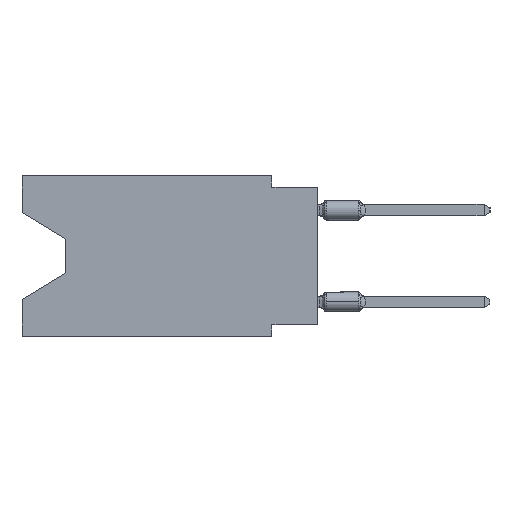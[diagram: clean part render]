
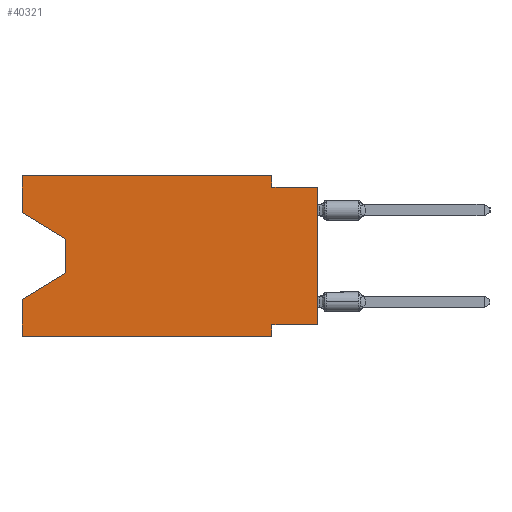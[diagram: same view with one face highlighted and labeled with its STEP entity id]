
A CAD part, left-side view. The second image highlights one B-rep face of the part: STEP entity #40321.
In plain terms, the highlighted planar face has unit normal (-1, 0, 0).
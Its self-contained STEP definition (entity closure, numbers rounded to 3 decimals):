
#712 = CARTESIAN_POINT ( 'NONE',  ( 0., 16.383, 0. ) ) ;
#977 = DIRECTION ( 'NONE',  ( 0., 0., 1. ) ) ;
#1176 = DIRECTION ( 'NONE',  ( 0., 0., -1. ) ) ;
#2780 = ORIENTED_EDGE ( 'NONE', *, *, #12342, .F. ) ;
#3453 = LINE ( 'NONE', #26692, #42703 ) ;
#3868 = CARTESIAN_POINT ( 'NONE',  ( 0., 13.97, -5.385 ) ) ;
#5465 = VERTEX_POINT ( 'NONE', #31540 ) ;
#5962 = VERTEX_POINT ( 'NONE', #16801 ) ;
#6063 = CARTESIAN_POINT ( 'NONE',  ( 0., 13.97, -3.505 ) ) ;
#6569 = LINE ( 'NONE', #40933, #33076 ) ;
#7921 = VECTOR ( 'NONE', #21574, 1000. ) ;
#8168 = DIRECTION ( 'NONE',  ( 0., -1., 0. ) ) ;
#9610 = VERTEX_POINT ( 'NONE', #15506 ) ;
#9838 = CARTESIAN_POINT ( 'NONE',  ( 0., 0., 0. ) ) ;
#9855 = DIRECTION ( 'NONE',  ( 0., 0., -1. ) ) ;
#9978 = LINE ( 'NONE', #25386, #7921 ) ;
#10222 = DIRECTION ( 'NONE',  ( 1., 0., 0. ) ) ;
#10704 = CARTESIAN_POINT ( 'NONE',  ( 0., 16.383, -8.89 ) ) ;
#11739 = VECTOR ( 'NONE', #8168, 1000. ) ;
#12045 = CARTESIAN_POINT ( 'NONE',  ( 0., 2.54, 0. ) ) ;
#12142 = CARTESIAN_POINT ( 'NONE',  ( 0., 16.383, -6.852 ) ) ;
#12342 = EDGE_CURVE ( 'NONE', #37248, #43170, #27362, .T. ) ;
#13881 = DIRECTION ( 'NONE',  ( 0., 0., 1. ) ) ;
#13892 = DIRECTION ( 'NONE',  ( 0., -0.855, -0.519 ) ) ;
#14019 = PLANE ( 'NONE',  #37804 ) ;
#14263 = FACE_OUTER_BOUND ( 'NONE', #23722, .T. ) ;
#14322 = EDGE_CURVE ( 'NONE', #17885, #20145, #6569, .T. ) ;
#14753 = ORIENTED_EDGE ( 'NONE', *, *, #25985, .T. ) ;
#15059 = EDGE_CURVE ( 'NONE', #43170, #9610, #46410, .T. ) ;
#15506 = CARTESIAN_POINT ( 'NONE',  ( 0., 2.54, -0.635 ) ) ;
#15628 = ORIENTED_EDGE ( 'NONE', *, *, #21421, .F. ) ;
#16246 = CARTESIAN_POINT ( 'NONE',  ( 0., 16.383, 0. ) ) ;
#16681 = DIRECTION ( 'NONE',  ( 0., 0., 1. ) ) ;
#16801 = CARTESIAN_POINT ( 'NONE',  ( 0., 16.383, -2.038 ) ) ;
#16958 = VECTOR ( 'NONE', #13892, 1000. ) ;
#17779 = LINE ( 'NONE', #10704, #24912 ) ;
#17885 = VERTEX_POINT ( 'NONE', #32952 ) ;
#18074 = EDGE_CURVE ( 'NONE', #42137, #5465, #17779, .T. ) ;
#19917 = LINE ( 'NONE', #712, #46518 ) ;
#20145 = VERTEX_POINT ( 'NONE', #23142 ) ;
#20218 = LINE ( 'NONE', #39437, #48343 ) ;
#20871 = ORIENTED_EDGE ( 'NONE', *, *, #38188, .F. ) ;
#21421 = EDGE_CURVE ( 'NONE', #9610, #41717, #26017, .T. ) ;
#21574 = DIRECTION ( 'NONE',  ( 0., 0.855, -0.519 ) ) ;
#21725 = CARTESIAN_POINT ( 'NONE',  ( 0., 2.54, 0. ) ) ;
#23142 = CARTESIAN_POINT ( 'NONE',  ( 0., 2.54, -8.255 ) ) ;
#23722 = EDGE_LOOP ( 'NONE', ( #14753, #25947, #23915, #25360, #29523, #34933, #33662, #35751, #15628, #30261, #2780, #20871 ) ) ;
#23915 = ORIENTED_EDGE ( 'NONE', *, *, #40317, .T. ) ;
#23977 = CARTESIAN_POINT ( 'NONE',  ( 0., 16.383, 0. ) ) ;
#24227 = VECTOR ( 'NONE', #1176, 1000. ) ;
#24912 = VECTOR ( 'NONE', #25862, 1000. ) ;
#25360 = ORIENTED_EDGE ( 'NONE', *, *, #40855, .F. ) ;
#25386 = CARTESIAN_POINT ( 'NONE',  ( 0., 13.97, -5.385 ) ) ;
#25634 = DIRECTION ( 'NONE',  ( 0., 0., -1. ) ) ;
#25741 = LINE ( 'NONE', #9838, #35634 ) ;
#25862 = DIRECTION ( 'NONE',  ( 0., -1., 0. ) ) ;
#25947 = ORIENTED_EDGE ( 'NONE', *, *, #44108, .T. ) ;
#25985 = EDGE_CURVE ( 'NONE', #5962, #43682, #48509, .T. ) ;
#26017 = LINE ( 'NONE', #41428, #28171 ) ;
#26259 = DIRECTION ( 'NONE',  ( 0., -1., 0. ) ) ;
#26644 = VECTOR ( 'NONE', #9855, 1000. ) ;
#26692 = CARTESIAN_POINT ( 'NONE',  ( 0., 2.54, -8.89 ) ) ;
#27362 = LINE ( 'NONE', #16246, #11739 ) ;
#28171 = VECTOR ( 'NONE', #26259, 1000. ) ;
#28269 = EDGE_CURVE ( 'NONE', #17885, #41717, #25741, .T. ) ;
#29307 = CARTESIAN_POINT ( 'NONE',  ( 0., 16.383, -2.038 ) ) ;
#29435 = CARTESIAN_POINT ( 'NONE',  ( 0., 16.383, 0. ) ) ;
#29523 = ORIENTED_EDGE ( 'NONE', *, *, #18074, .T. ) ;
#30261 = ORIENTED_EDGE ( 'NONE', *, *, #15059, .F. ) ;
#31540 = CARTESIAN_POINT ( 'NONE',  ( 0., 2.54, -8.89 ) ) ;
#32436 = CARTESIAN_POINT ( 'NONE',  ( 0., 0., -0.635 ) ) ;
#32952 = CARTESIAN_POINT ( 'NONE',  ( 0., 0., -8.255 ) ) ;
#33076 = VECTOR ( 'NONE', #33368, 1000. ) ;
#33368 = DIRECTION ( 'NONE',  ( 0., 1., 0. ) ) ;
#33662 = ORIENTED_EDGE ( 'NONE', *, *, #14322, .F. ) ;
#34933 = ORIENTED_EDGE ( 'NONE', *, *, #41617, .F. ) ;
#35634 = VECTOR ( 'NONE', #13881, 1000. ) ;
#35751 = ORIENTED_EDGE ( 'NONE', *, *, #28269, .T. ) ;
#37248 = VERTEX_POINT ( 'NONE', #23977 ) ;
#37804 = AXIS2_PLACEMENT_3D ( 'NONE', #29435, #10222, #25634 ) ;
#38188 = EDGE_CURVE ( 'NONE', #5962, #37248, #19917, .T. ) ;
#39437 = CARTESIAN_POINT ( 'NONE',  ( 0., 16.383, 0. ) ) ;
#40317 = EDGE_CURVE ( 'NONE', #44621, #47101, #9978, .T. ) ;
#40321 = ADVANCED_FACE ( 'NONE', ( #14263 ), #14019, .F. ) ;
#40855 = EDGE_CURVE ( 'NONE', #42137, #47101, #20218, .T. ) ;
#40933 = CARTESIAN_POINT ( 'NONE',  ( 0., 0., -8.255 ) ) ;
#41428 = CARTESIAN_POINT ( 'NONE',  ( 0., 0., -0.635 ) ) ;
#41613 = DIRECTION ( 'NONE',  ( 0., 0., -1. ) ) ;
#41617 = EDGE_CURVE ( 'NONE', #20145, #5465, #3453, .T. ) ;
#41717 = VERTEX_POINT ( 'NONE', #32436 ) ;
#42137 = VERTEX_POINT ( 'NONE', #49704 ) ;
#42703 = VECTOR ( 'NONE', #41613, 1000. ) ;
#43170 = VERTEX_POINT ( 'NONE', #21725 ) ;
#43682 = VERTEX_POINT ( 'NONE', #46725 ) ;
#44108 = EDGE_CURVE ( 'NONE', #43682, #44621, #44477, .T. ) ;
#44477 = LINE ( 'NONE', #6063, #26644 ) ;
#44621 = VERTEX_POINT ( 'NONE', #3868 ) ;
#46410 = LINE ( 'NONE', #12045, #24227 ) ;
#46518 = VECTOR ( 'NONE', #977, 1000. ) ;
#46725 = CARTESIAN_POINT ( 'NONE',  ( 0., 13.97, -3.505 ) ) ;
#47101 = VERTEX_POINT ( 'NONE', #12142 ) ;
#48343 = VECTOR ( 'NONE', #16681, 1000. ) ;
#48509 = LINE ( 'NONE', #29307, #16958 ) ;
#49704 = CARTESIAN_POINT ( 'NONE',  ( 0., 16.383, -8.89 ) ) ;
